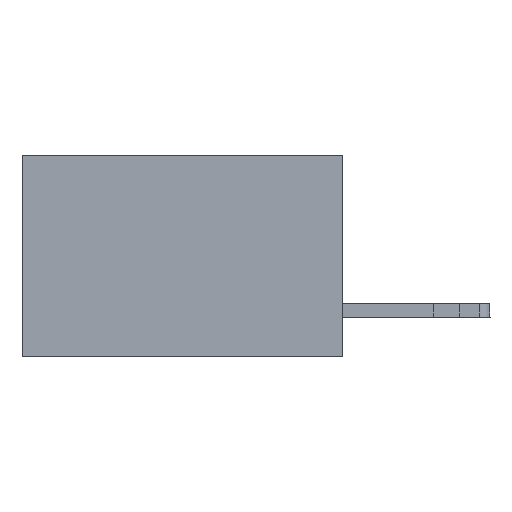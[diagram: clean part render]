
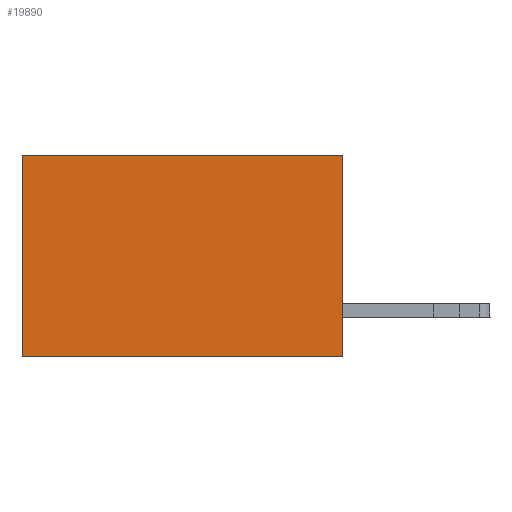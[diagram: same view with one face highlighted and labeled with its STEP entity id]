
A CAD part, left-side view. The second image highlights one B-rep face of the part: STEP entity #19890.
In plain terms, the highlighted planar face has unit normal (-1, 0, 0).
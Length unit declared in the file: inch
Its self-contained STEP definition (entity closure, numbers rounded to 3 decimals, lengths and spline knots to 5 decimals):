
#412 = LINE ( 'NONE', #18883, #1050 ) ;
#442 = VERTEX_POINT ( 'NONE', #3539 ) ;
#1050 = VECTOR ( 'NONE', #18850, 39.37008 ) ;
#1586 = ORIENTED_EDGE ( 'NONE', *, *, #18244, .F. ) ;
#3539 = CARTESIAN_POINT ( 'NONE',  ( 0.277, 0., -0.37 ) ) ;
#4036 = LINE ( 'NONE', #16352, #14022 ) ;
#4471 = VECTOR ( 'NONE', #5561, 39.37008 ) ;
#4785 = EDGE_CURVE ( 'NONE', #16509, #21093, #412, .T. ) ;
#5561 = DIRECTION ( 'NONE',  ( 0., 0., -1. ) ) ;
#7028 = LINE ( 'NONE', #17371, #17004 ) ;
#8146 = ORIENTED_EDGE ( 'NONE', *, *, #17439, .T. ) ;
#8469 = FACE_OUTER_BOUND ( 'NONE', #18190, .T. ) ;
#8762 = CARTESIAN_POINT ( 'NONE',  ( 0.277, 0., -0.37 ) ) ;
#9402 = DIRECTION ( 'NONE',  ( 0., 1., 0. ) ) ;
#10774 = DIRECTION ( 'NONE',  ( 1., 0., 0. ) ) ;
#10924 = ORIENTED_EDGE ( 'NONE', *, *, #4785, .T. ) ;
#11548 = CARTESIAN_POINT ( 'NONE',  ( 0.277, 0.59, 0. ) ) ;
#11744 = AXIS2_PLACEMENT_3D ( 'NONE', #8762, #10774, #24602 ) ;
#12173 = ORIENTED_EDGE ( 'NONE', *, *, #19023, .F. ) ;
#13170 = VERTEX_POINT ( 'NONE', #14739 ) ;
#14022 = VECTOR ( 'NONE', #22193, 39.37008 ) ;
#14143 = CARTESIAN_POINT ( 'NONE',  ( 0.277, 0.59, -0.37 ) ) ;
#14739 = CARTESIAN_POINT ( 'NONE',  ( 0.277, 0., 0. ) ) ;
#16352 = CARTESIAN_POINT ( 'NONE',  ( 0.277, 0., 0. ) ) ;
#16509 = VERTEX_POINT ( 'NONE', #11548 ) ;
#17004 = VECTOR ( 'NONE', #9402, 39.37008 ) ;
#17371 = CARTESIAN_POINT ( 'NONE',  ( 0.277, 0., -0.37 ) ) ;
#17439 = EDGE_CURVE ( 'NONE', #13170, #16509, #4036, .T. ) ;
#17503 = CARTESIAN_POINT ( 'NONE',  ( 0.277, 0., -0.37 ) ) ;
#18190 = EDGE_LOOP ( 'NONE', ( #10924, #1586, #12173, #8146 ) ) ;
#18244 = EDGE_CURVE ( 'NONE', #442, #21093, #7028, .T. ) ;
#18850 = DIRECTION ( 'NONE',  ( 0., 0., -1. ) ) ;
#18883 = CARTESIAN_POINT ( 'NONE',  ( 0.277, 0.59, -0.37 ) ) ;
#19023 = EDGE_CURVE ( 'NONE', #13170, #442, #20352, .T. ) ;
#19890 = ADVANCED_FACE ( 'NONE', ( #8469 ), #22630, .F. ) ;
#20352 = LINE ( 'NONE', #17503, #4471 ) ;
#21093 = VERTEX_POINT ( 'NONE', #14143 ) ;
#22193 = DIRECTION ( 'NONE',  ( 0., 1., 0. ) ) ;
#22630 = PLANE ( 'NONE',  #11744 ) ;
#24602 = DIRECTION ( 'NONE',  ( 0., 0., -1. ) ) ;
